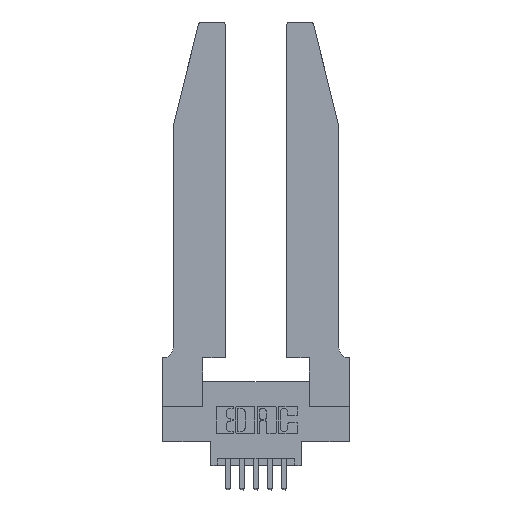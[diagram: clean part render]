
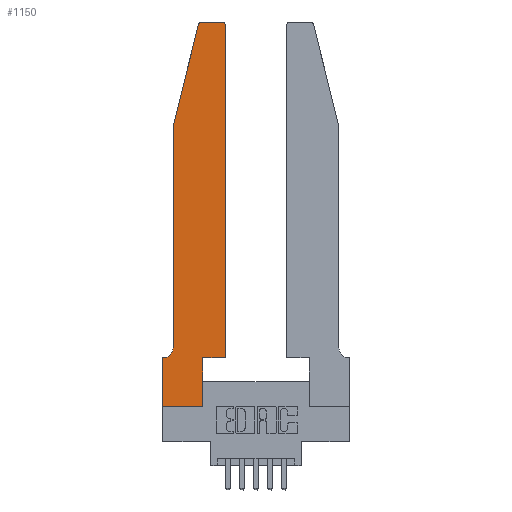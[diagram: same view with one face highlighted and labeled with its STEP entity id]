
A CAD part, top view. The second image highlights one B-rep face of the part: STEP entity #1150.
In plain terms, the highlighted planar face has unit normal (0, 0, 1).
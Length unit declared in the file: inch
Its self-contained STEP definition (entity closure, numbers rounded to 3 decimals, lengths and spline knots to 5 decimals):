
#167 = LINE ( 'NONE', #11444, #3716 ) ;
#305 = ORIENTED_EDGE ( 'NONE', *, *, #3352, .T. ) ;
#429 = VERTEX_POINT ( 'NONE', #12605 ) ;
#530 = CIRCLE ( 'NONE', #13144, 0.03 ) ;
#551 = CARTESIAN_POINT ( 'NONE',  ( 0.0055, 0.42, 0.37 ) ) ;
#853 = CARTESIAN_POINT ( 'NONE',  ( 0.4505, 0.35, 0.37 ) ) ;
#953 = DIRECTION ( 'NONE',  ( -1., 0., 0. ) ) ;
#1150 = ADVANCED_FACE ( 'NONE', ( #8574 ), #11083, .T. ) ;
#1267 = CARTESIAN_POINT ( 'NONE',  ( 0., 0., 0.37 ) ) ;
#1361 = EDGE_CURVE ( 'NONE', #2852, #5089, #530, .T. ) ;
#1660 = DIRECTION ( 'NONE',  ( -1., 0., 0. ) ) ;
#1673 = AXIS2_PLACEMENT_3D ( 'NONE', #9858, #13035, #8148 ) ;
#1681 = VECTOR ( 'NONE', #8434, 39.37008 ) ;
#1687 = DIRECTION ( 'NONE',  ( 0., 1., 0. ) ) ;
#1709 = LINE ( 'NONE', #11304, #12737 ) ;
#2315 = EDGE_CURVE ( 'NONE', #5757, #6348, #13263, .T. ) ;
#2317 = VERTEX_POINT ( 'NONE', #853 ) ;
#2547 = DIRECTION ( 'NONE',  ( 0., 1., 0. ) ) ;
#2701 = ORIENTED_EDGE ( 'NONE', *, *, #13215, .T. ) ;
#2852 = VERTEX_POINT ( 'NONE', #7767 ) ;
#2946 = CARTESIAN_POINT ( 'NONE',  ( 0.0755, 2., 0.37 ) ) ;
#3025 = EDGE_CURVE ( 'NONE', #6396, #12336, #167, .T. ) ;
#3312 = EDGE_CURVE ( 'NONE', #9267, #2317, #7859, .T. ) ;
#3331 = CARTESIAN_POINT ( 'NONE',  ( 0.4505, 0.35, 0.37 ) ) ;
#3352 = EDGE_CURVE ( 'NONE', #5050, #10827, #12536, .T. ) ;
#3520 = CARTESIAN_POINT ( 'NONE',  ( 0., 0., 0.37 ) ) ;
#3537 = ORIENTED_EDGE ( 'NONE', *, *, #12789, .T. ) ;
#3716 = VECTOR ( 'NONE', #12764, 39.37008 ) ;
#3831 = LINE ( 'NONE', #3331, #6676 ) ;
#4031 = ORIENTED_EDGE ( 'NONE', *, *, #11044, .T. ) ;
#4204 = ORIENTED_EDGE ( 'NONE', *, *, #3025, .T. ) ;
#4238 = EDGE_CURVE ( 'NONE', #2317, #2852, #3831, .T. ) ;
#4383 = ORIENTED_EDGE ( 'NONE', *, *, #4238, .T. ) ;
#4406 = CIRCLE ( 'NONE', #8775, 0.07 ) ;
#4559 = DIRECTION ( 'NONE',  ( 0., -1., 0. ) ) ;
#4566 = DIRECTION ( 'NONE',  ( 1., 0., 0. ) ) ;
#4584 = DIRECTION ( 'NONE',  ( 0., 0., 1. ) ) ;
#4655 = CARTESIAN_POINT ( 'NONE',  ( 0.2865, 0.35, 0.37 ) ) ;
#4717 = VECTOR ( 'NONE', #13160, 39.37008 ) ;
#5050 = VERTEX_POINT ( 'NONE', #5516 ) ;
#5089 = VERTEX_POINT ( 'NONE', #11924 ) ;
#5219 = VECTOR ( 'NONE', #953, 39.37008 ) ;
#5516 = CARTESIAN_POINT ( 'NONE',  ( 0.284, 2.75, 0.37 ) ) ;
#5554 = ORIENTED_EDGE ( 'NONE', *, *, #2315, .T. ) ;
#5757 = VERTEX_POINT ( 'NONE', #12218 ) ;
#5879 = ORIENTED_EDGE ( 'NONE', *, *, #7534, .T. ) ;
#6126 = CARTESIAN_POINT ( 'NONE',  ( 0.284, 2.72, 0.37 ) ) ;
#6256 = CARTESIAN_POINT ( 'NONE',  ( 0.4505, 0.35, 0.37 ) ) ;
#6348 = VERTEX_POINT ( 'NONE', #8186 ) ;
#6396 = VERTEX_POINT ( 'NONE', #2946 ) ;
#6676 = VECTOR ( 'NONE', #2547, 39.37008 ) ;
#6749 = DIRECTION ( 'NONE',  ( -1., 0., 0. ) ) ;
#6873 = ORIENTED_EDGE ( 'NONE', *, *, #3312, .T. ) ;
#7281 = EDGE_LOOP ( 'NONE', ( #13924, #305, #3537, #4204, #7360, #2701, #5554, #5879, #4031, #6873, #4383, #7542 ) ) ;
#7328 = CARTESIAN_POINT ( 'NONE',  ( 0.0755, 2., 0.37 ) ) ;
#7360 = ORIENTED_EDGE ( 'NONE', *, *, #12082, .T. ) ;
#7534 = EDGE_CURVE ( 'NONE', #6348, #9782, #13822, .T. ) ;
#7542 = ORIENTED_EDGE ( 'NONE', *, *, #1361, .T. ) ;
#7566 = VECTOR ( 'NONE', #4559, 39.37008 ) ;
#7767 = CARTESIAN_POINT ( 'NONE',  ( 0.4505, 2.72, 0.37 ) ) ;
#7859 = LINE ( 'NONE', #6256, #4717 ) ;
#7878 = VECTOR ( 'NONE', #6749, 39.37008 ) ;
#7895 = CARTESIAN_POINT ( 'NONE',  ( 0.4205, 2.72, 0.37 ) ) ;
#8046 = DIRECTION ( 'NONE',  ( 0., 0., -1. ) ) ;
#8148 = DIRECTION ( 'NONE',  ( 1., 0., 0. ) ) ;
#8186 = CARTESIAN_POINT ( 'NONE',  ( 0., 0., 0.37 ) ) ;
#8340 = LINE ( 'NONE', #10530, #5219 ) ;
#8434 = DIRECTION ( 'NONE',  ( -0.239, -0.971, 0. ) ) ;
#8574 = FACE_OUTER_BOUND ( 'NONE', #7281, .T. ) ;
#8657 = AXIS2_PLACEMENT_3D ( 'NONE', #6126, #4584, #4566 ) ;
#8734 = DIRECTION ( 'NONE',  ( 0., 0., 1. ) ) ;
#8775 = AXIS2_PLACEMENT_3D ( 'NONE', #551, #8046, #1660 ) ;
#8826 = CARTESIAN_POINT ( 'NONE',  ( 0.25487, 2.72718, 0.37 ) ) ;
#8901 = CARTESIAN_POINT ( 'NONE',  ( 0.2865, 0., 0.37 ) ) ;
#9255 = EDGE_CURVE ( 'NONE', #5089, #5050, #10723, .T. ) ;
#9267 = VERTEX_POINT ( 'NONE', #4655 ) ;
#9451 = CARTESIAN_POINT ( 'NONE',  ( 0.0755, 0.42, 0.37 ) ) ;
#9782 = VERTEX_POINT ( 'NONE', #8901 ) ;
#9820 = DIRECTION ( 'NONE',  ( 1., 0., 0. ) ) ;
#9858 = CARTESIAN_POINT ( 'NONE',  ( 0., 0.35, 0.37 ) ) ;
#10530 = CARTESIAN_POINT ( 'NONE',  ( 0.0755, 0.35, 0.37 ) ) ;
#10723 = LINE ( 'NONE', #10987, #7878 ) ;
#10827 = VERTEX_POINT ( 'NONE', #8826 ) ;
#10886 = DIRECTION ( 'NONE',  ( 1., 0., 0. ) ) ;
#10987 = CARTESIAN_POINT ( 'NONE',  ( 0.2605, 2.75, 0.37 ) ) ;
#11044 = EDGE_CURVE ( 'NONE', #9782, #9267, #1709, .T. ) ;
#11083 = PLANE ( 'NONE',  #1673 ) ;
#11268 = VECTOR ( 'NONE', #9820, 39.37008 ) ;
#11304 = CARTESIAN_POINT ( 'NONE',  ( 0.2865, 0.35, 0.37 ) ) ;
#11444 = CARTESIAN_POINT ( 'NONE',  ( 0.0755, 2., 0.37 ) ) ;
#11924 = CARTESIAN_POINT ( 'NONE',  ( 0.4205, 2.75, 0.37 ) ) ;
#12082 = EDGE_CURVE ( 'NONE', #12336, #429, #4406, .T. ) ;
#12218 = CARTESIAN_POINT ( 'NONE',  ( 0., 0.35, 0.37 ) ) ;
#12336 = VERTEX_POINT ( 'NONE', #9451 ) ;
#12536 = CIRCLE ( 'NONE', #8657, 0.03 ) ;
#12605 = CARTESIAN_POINT ( 'NONE',  ( 0.0055, 0.35, 0.37 ) ) ;
#12737 = VECTOR ( 'NONE', #1687, 39.37008 ) ;
#12764 = DIRECTION ( 'NONE',  ( 0., -1., 0. ) ) ;
#12789 = EDGE_CURVE ( 'NONE', #10827, #6396, #13059, .T. ) ;
#13035 = DIRECTION ( 'NONE',  ( 0., 0., 1. ) ) ;
#13059 = LINE ( 'NONE', #7328, #1681 ) ;
#13144 = AXIS2_PLACEMENT_3D ( 'NONE', #7895, #8734, #10886 ) ;
#13160 = DIRECTION ( 'NONE',  ( 1., 0., 0. ) ) ;
#13215 = EDGE_CURVE ( 'NONE', #429, #5757, #8340, .T. ) ;
#13263 = LINE ( 'NONE', #3520, #7566 ) ;
#13822 = LINE ( 'NONE', #1267, #11268 ) ;
#13924 = ORIENTED_EDGE ( 'NONE', *, *, #9255, .T. ) ;
